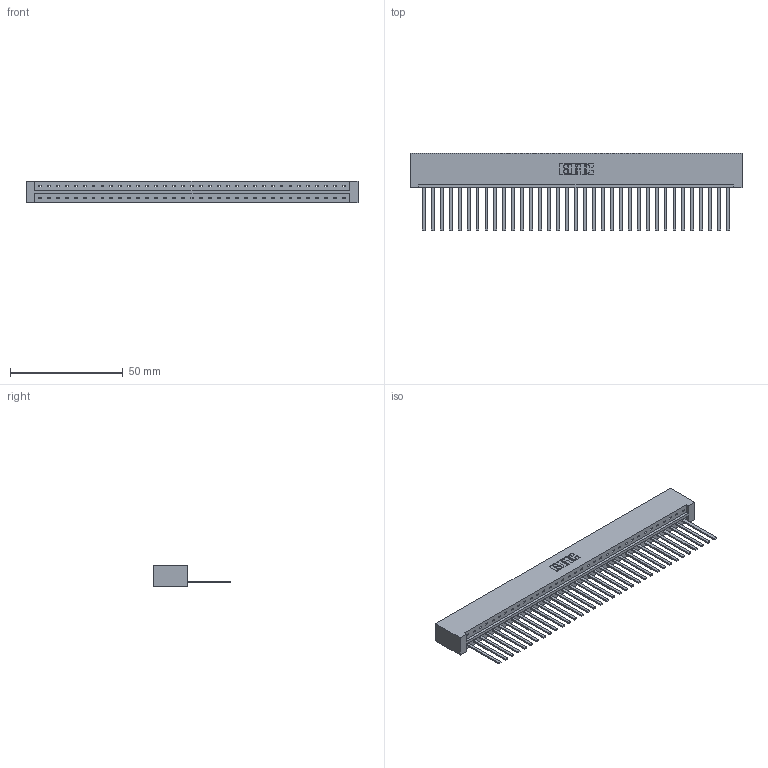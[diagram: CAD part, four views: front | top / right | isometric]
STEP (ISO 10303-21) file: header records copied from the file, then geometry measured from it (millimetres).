
FILE_DESCRIPTION (( 'STEP AP203' ), '1' );
FILE_NAME ('833-035-544-101.STEP', '2020-06-03T00:56:00', ( '' ), ( '' ), 'SwSTEP 2.0', 'SolidWorks 2020', '' );
FILE_SCHEMA (( 'CONFIG_CONTROL_DESIGN' ));
Length unit declared in the file: inch
Products named in the file (3): 345-292-001_345-293-144; 833 Part_Lugless; 833-035-544-101
Assembly tree (36 placements, depth 2):
  833-035-544-101
    833 Part_Lugless
    345-292-001_345-293-144  x35
Bounding box: 146.94 x 34.3 x 9.4 mm (x, y, z)
Volume: 15744.1 mm3; surface area: 18263.6 mm2
Topology: 36 solids, 36 shells, 1926 faces, 5817 edges, 3830 vertices
Faces by surface type: plane 1396, cylinder 530
Entity records: 21841 total; most frequent: CARTESIAN_POINT 3775, ORIENTED_EDGE 3746, DIRECTION 3187, EDGE_CURVE 1873, LINE 1757, VECTOR 1757, VERTEX_POINT 1246, AXIS2_PLACEMENT_3D 715
